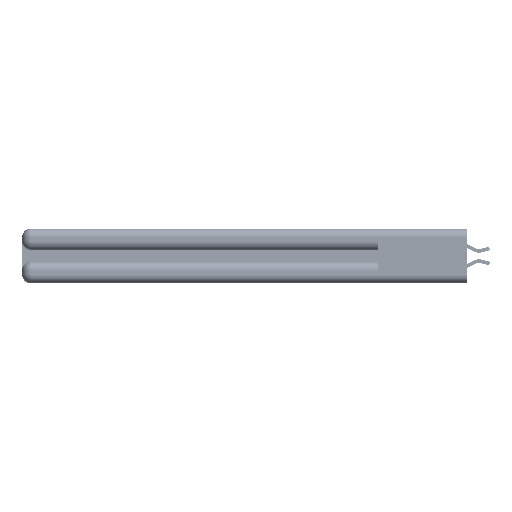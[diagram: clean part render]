
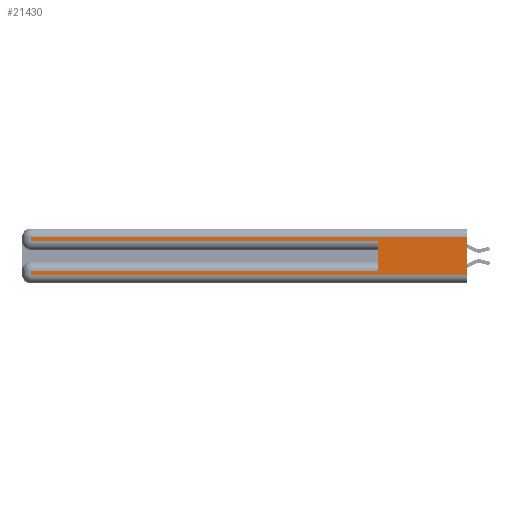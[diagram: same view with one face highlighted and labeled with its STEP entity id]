
A CAD part, left-side view. The second image highlights one B-rep face of the part: STEP entity #21430.
In plain terms, the highlighted planar face has unit normal (-1, 0, 0).
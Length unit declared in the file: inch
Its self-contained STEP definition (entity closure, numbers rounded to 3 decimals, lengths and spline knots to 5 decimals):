
#34 = EDGE_LOOP ( 'NONE', ( #17867, #47792, #20259, #21442, #12567, #13751, #4839, #17316 ) ) ;
#107 = AXIS2_PLACEMENT_3D ( 'NONE', #39532, #20901, #47089 ) ;
#595 = VERTEX_POINT ( 'NONE', #25068 ) ;
#1809 = EDGE_CURVE ( 'NONE', #21768, #39869, #33857, .T. ) ;
#2149 = EDGE_CURVE ( 'NONE', #14845, #20941, #48487, .T. ) ;
#4080 = EDGE_CURVE ( 'NONE', #28924, #595, #14857, .T. ) ;
#4484 = VERTEX_POINT ( 'NONE', #43111 ) ;
#4839 = ORIENTED_EDGE ( 'NONE', *, *, #1809, .T. ) ;
#5698 = LINE ( 'NONE', #38330, #13423 ) ;
#6321 = DIRECTION ( 'NONE',  ( 0., 0., -1. ) ) ;
#6581 = DIRECTION ( 'NONE',  ( 0., 1., 0. ) ) ;
#7064 = VECTOR ( 'NONE', #6581, 39.37008 ) ;
#8964 = CARTESIAN_POINT ( 'NONE',  ( 0., 2.94, 0.31 ) ) ;
#10812 = CARTESIAN_POINT ( 'NONE',  ( 0., 0.6, 0.145 ) ) ;
#11675 = EDGE_CURVE ( 'NONE', #20941, #595, #44800, .T. ) ;
#12567 = ORIENTED_EDGE ( 'NONE', *, *, #4080, .F. ) ;
#13423 = VECTOR ( 'NONE', #15874, 39.37008 ) ;
#13691 = VECTOR ( 'NONE', #40816, 39.37008 ) ;
#13751 = ORIENTED_EDGE ( 'NONE', *, *, #39818, .T. ) ;
#14267 = VECTOR ( 'NONE', #22865, 39.37008 ) ;
#14845 = VERTEX_POINT ( 'NONE', #8964 ) ;
#14857 = LINE ( 'NONE', #10812, #13691 ) ;
#15034 = VECTOR ( 'NONE', #15783, 39.37008 ) ;
#15783 = DIRECTION ( 'NONE',  ( 0., 0., -1. ) ) ;
#15874 = DIRECTION ( 'NONE',  ( 0., 1., 0. ) ) ;
#15932 = CARTESIAN_POINT ( 'NONE',  ( 0., 0., 0.285 ) ) ;
#16347 = FACE_OUTER_BOUND ( 'NONE', #34, .T. ) ;
#17104 = PLANE ( 'NONE',  #107 ) ;
#17316 = ORIENTED_EDGE ( 'NONE', *, *, #19834, .T. ) ;
#17867 = ORIENTED_EDGE ( 'NONE', *, *, #38784, .F. ) ;
#19742 = DIRECTION ( 'NONE',  ( 0., -1., 0. ) ) ;
#19834 = EDGE_CURVE ( 'NONE', #39869, #37255, #29462, .T. ) ;
#20259 = ORIENTED_EDGE ( 'NONE', *, *, #2149, .T. ) ;
#20901 = DIRECTION ( 'NONE',  ( 1., 0., 0. ) ) ;
#20941 = VERTEX_POINT ( 'NONE', #40544 ) ;
#21430 = ADVANCED_FACE ( 'NONE', ( #16347 ), #17104, .F. ) ;
#21442 = ORIENTED_EDGE ( 'NONE', *, *, #11675, .T. ) ;
#21768 = VERTEX_POINT ( 'NONE', #26758 ) ;
#22865 = DIRECTION ( 'NONE',  ( 0., 0., -1. ) ) ;
#24895 = VECTOR ( 'NONE', #19742, 39.37008 ) ;
#25068 = CARTESIAN_POINT ( 'NONE',  ( 0., 0.6, 0.285 ) ) ;
#25736 = CARTESIAN_POINT ( 'NONE',  ( 0., 2.94, 0.06 ) ) ;
#26598 = DIRECTION ( 'NONE',  ( 0., -1., 0. ) ) ;
#26758 = CARTESIAN_POINT ( 'NONE',  ( 0., 2.94, 0.085 ) ) ;
#28756 = CARTESIAN_POINT ( 'NONE',  ( 0., 2.94, 0.37 ) ) ;
#28924 = VERTEX_POINT ( 'NONE', #38911 ) ;
#29462 = LINE ( 'NONE', #45221, #31837 ) ;
#31837 = VECTOR ( 'NONE', #26598, 39.37008 ) ;
#33857 = LINE ( 'NONE', #34336, #15034 ) ;
#34336 = CARTESIAN_POINT ( 'NONE',  ( 0., 2.94, 0.37 ) ) ;
#35646 = EDGE_CURVE ( 'NONE', #4484, #14845, #5698, .T. ) ;
#36878 = CARTESIAN_POINT ( 'NONE',  ( 0., 0., 0.06 ) ) ;
#37054 = LINE ( 'NONE', #44055, #7064 ) ;
#37255 = VERTEX_POINT ( 'NONE', #36878 ) ;
#38330 = CARTESIAN_POINT ( 'NONE',  ( 0., 0., 0.31 ) ) ;
#38486 = VECTOR ( 'NONE', #6321, 39.37008 ) ;
#38784 = EDGE_CURVE ( 'NONE', #4484, #37255, #43044, .T. ) ;
#38911 = CARTESIAN_POINT ( 'NONE',  ( 0., 0.6, 0.085 ) ) ;
#39532 = CARTESIAN_POINT ( 'NONE',  ( 0., 0., 0.37 ) ) ;
#39818 = EDGE_CURVE ( 'NONE', #28924, #21768, #37054, .T. ) ;
#39869 = VERTEX_POINT ( 'NONE', #25736 ) ;
#40544 = CARTESIAN_POINT ( 'NONE',  ( 0., 2.94, 0.285 ) ) ;
#40816 = DIRECTION ( 'NONE',  ( 0., 0., 1. ) ) ;
#43044 = LINE ( 'NONE', #45277, #14267 ) ;
#43111 = CARTESIAN_POINT ( 'NONE',  ( 0., 0., 0.31 ) ) ;
#44055 = CARTESIAN_POINT ( 'NONE',  ( 0., 0., 0.085 ) ) ;
#44800 = LINE ( 'NONE', #15932, #24895 ) ;
#45221 = CARTESIAN_POINT ( 'NONE',  ( 0., 0., 0.06 ) ) ;
#45277 = CARTESIAN_POINT ( 'NONE',  ( 0., 0., 0.37 ) ) ;
#47089 = DIRECTION ( 'NONE',  ( 0., 0., -1. ) ) ;
#47792 = ORIENTED_EDGE ( 'NONE', *, *, #35646, .T. ) ;
#48487 = LINE ( 'NONE', #28756, #38486 ) ;
